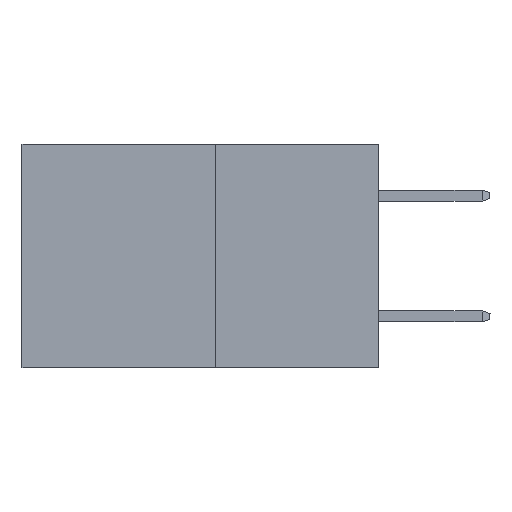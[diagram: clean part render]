
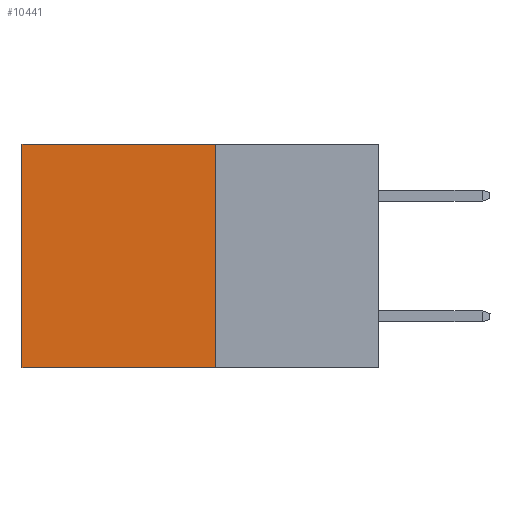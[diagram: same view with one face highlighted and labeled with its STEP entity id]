
A CAD part, left-side view. The second image highlights one B-rep face of the part: STEP entity #10441.
In plain terms, the highlighted planar face has unit normal (-1, 0, 0).
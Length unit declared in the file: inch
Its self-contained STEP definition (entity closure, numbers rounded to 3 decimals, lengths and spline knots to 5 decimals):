
#160 = CARTESIAN_POINT ( 'NONE',  ( 0.277, 0.27, -0.37 ) ) ;
#476 = CARTESIAN_POINT ( 'NONE',  ( 0.277, 0.59, 0. ) ) ;
#495 = CARTESIAN_POINT ( 'NONE',  ( 0.277, 0.27, -0.37 ) ) ;
#1094 = DIRECTION ( 'NONE',  ( 1., 0., 0. ) ) ;
#1111 = VERTEX_POINT ( 'NONE', #6757 ) ;
#1487 = EDGE_CURVE ( 'NONE', #4623, #3826, #7118, .T. ) ;
#1800 = LINE ( 'NONE', #5360, #8254 ) ;
#1918 = CARTESIAN_POINT ( 'NONE',  ( 0.277, 0.27, 0. ) ) ;
#1941 = DIRECTION ( 'NONE',  ( 0., 1., 0. ) ) ;
#2321 = EDGE_LOOP ( 'NONE', ( #9159, #9144, #9094, #8984 ) ) ;
#2343 = EDGE_CURVE ( 'NONE', #10056, #3826, #1800, .T. ) ;
#3590 = LINE ( 'NONE', #9791, #5056 ) ;
#3826 = VERTEX_POINT ( 'NONE', #4132 ) ;
#4132 = CARTESIAN_POINT ( 'NONE',  ( 0.277, 0.59, -0.37 ) ) ;
#4155 = LINE ( 'NONE', #1918, #10988 ) ;
#4623 = VERTEX_POINT ( 'NONE', #476 ) ;
#5000 = VECTOR ( 'NONE', #7658, 39.37008 ) ;
#5056 = VECTOR ( 'NONE', #9802, 39.37008 ) ;
#5138 = EDGE_CURVE ( 'NONE', #1111, #10056, #3590, .T. ) ;
#5360 = CARTESIAN_POINT ( 'NONE',  ( 0.277, 0.27, -0.37 ) ) ;
#5481 = PLANE ( 'NONE',  #5621 ) ;
#5621 = AXIS2_PLACEMENT_3D ( 'NONE', #160, #1094, #7073 ) ;
#6629 = EDGE_CURVE ( 'NONE', #1111, #4623, #4155, .T. ) ;
#6757 = CARTESIAN_POINT ( 'NONE',  ( 0.277, 0.27, 0. ) ) ;
#7073 = DIRECTION ( 'NONE',  ( 0., 0., -1. ) ) ;
#7118 = LINE ( 'NONE', #9931, #5000 ) ;
#7658 = DIRECTION ( 'NONE',  ( 0., 0., -1. ) ) ;
#8254 = VECTOR ( 'NONE', #8349, 39.37008 ) ;
#8349 = DIRECTION ( 'NONE',  ( 0., 1., 0. ) ) ;
#8374 = FACE_OUTER_BOUND ( 'NONE', #2321, .T. ) ;
#8984 = ORIENTED_EDGE ( 'NONE', *, *, #6629, .T. ) ;
#9094 = ORIENTED_EDGE ( 'NONE', *, *, #5138, .F. ) ;
#9144 = ORIENTED_EDGE ( 'NONE', *, *, #2343, .F. ) ;
#9159 = ORIENTED_EDGE ( 'NONE', *, *, #1487, .T. ) ;
#9791 = CARTESIAN_POINT ( 'NONE',  ( 0.277, 0.27, -0.37 ) ) ;
#9802 = DIRECTION ( 'NONE',  ( 0., 0., -1. ) ) ;
#9931 = CARTESIAN_POINT ( 'NONE',  ( 0.277, 0.59, -0.37 ) ) ;
#10056 = VERTEX_POINT ( 'NONE', #495 ) ;
#10441 = ADVANCED_FACE ( 'NONE', ( #8374 ), #5481, .F. ) ;
#10988 = VECTOR ( 'NONE', #1941, 39.37008 ) ;
